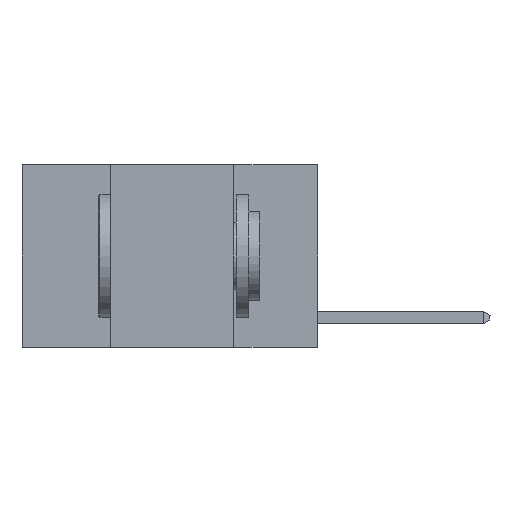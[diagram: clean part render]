
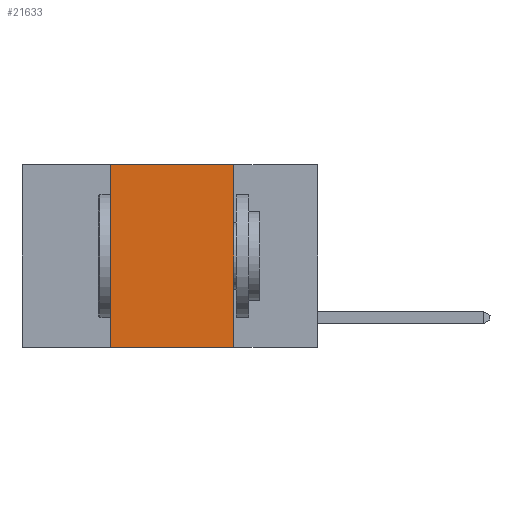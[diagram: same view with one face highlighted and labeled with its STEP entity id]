
A CAD part, left-side view. The second image highlights one B-rep face of the part: STEP entity #21633.
In plain terms, the highlighted planar face has unit normal (-1, 0, 0).
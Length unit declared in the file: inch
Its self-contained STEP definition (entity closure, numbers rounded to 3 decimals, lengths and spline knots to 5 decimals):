
#229 = CARTESIAN_POINT ( 'NONE',  ( 0., 0.17, 0. ) ) ;
#796 = DIRECTION ( 'NONE',  ( 1., 0., 0. ) ) ;
#931 = DIRECTION ( 'NONE',  ( 0., 0., -1. ) ) ;
#1075 = CARTESIAN_POINT ( 'NONE',  ( 0., 0.42, 0. ) ) ;
#3218 = CARTESIAN_POINT ( 'NONE',  ( 0., 0.17, -0.37 ) ) ;
#4366 = FACE_OUTER_BOUND ( 'NONE', #9969, .T. ) ;
#5682 = AXIS2_PLACEMENT_3D ( 'NONE', #17967, #796, #931 ) ;
#6763 = CARTESIAN_POINT ( 'NONE',  ( 0., 0.42, -0.37 ) ) ;
#7864 = CARTESIAN_POINT ( 'NONE',  ( 0., 0.42, 0. ) ) ;
#9466 = CARTESIAN_POINT ( 'NONE',  ( 0., 0.6, 0. ) ) ;
#9570 = EDGE_CURVE ( 'NONE', #17184, #23157, #17550, .T. ) ;
#9969 = EDGE_LOOP ( 'NONE', ( #13974, #13538, #19743, #16135 ) ) ;
#11245 = VECTOR ( 'NONE', #22871, 39.37008 ) ;
#11445 = DIRECTION ( 'NONE',  ( 0., 0., 1. ) ) ;
#12178 = LINE ( 'NONE', #13918, #15008 ) ;
#12338 = DIRECTION ( 'NONE',  ( 0., 0., -1. ) ) ;
#12817 = VERTEX_POINT ( 'NONE', #3218 ) ;
#13538 = ORIENTED_EDGE ( 'NONE', *, *, #23262, .F. ) ;
#13715 = EDGE_CURVE ( 'NONE', #22496, #12817, #23728, .T. ) ;
#13873 = PLANE ( 'NONE',  #5682 ) ;
#13918 = CARTESIAN_POINT ( 'NONE',  ( 0., 0.6, -0.37 ) ) ;
#13974 = ORIENTED_EDGE ( 'NONE', *, *, #13715, .F. ) ;
#15008 = VECTOR ( 'NONE', #21244, 39.37008 ) ;
#15680 = LINE ( 'NONE', #9466, #11245 ) ;
#15823 = VECTOR ( 'NONE', #12338, 39.37008 ) ;
#16135 = ORIENTED_EDGE ( 'NONE', *, *, #17335, .T. ) ;
#17184 = VERTEX_POINT ( 'NONE', #6763 ) ;
#17335 = EDGE_CURVE ( 'NONE', #17184, #12817, #12178, .T. ) ;
#17550 = LINE ( 'NONE', #7864, #23954 ) ;
#17967 = CARTESIAN_POINT ( 'NONE',  ( 0., 0.6, 0. ) ) ;
#18043 = CARTESIAN_POINT ( 'NONE',  ( 0., 0.17, 0. ) ) ;
#19743 = ORIENTED_EDGE ( 'NONE', *, *, #9570, .F. ) ;
#21244 = DIRECTION ( 'NONE',  ( 0., -1., 0. ) ) ;
#21633 = ADVANCED_FACE ( 'NONE', ( #4366 ), #13873, .F. ) ;
#22496 = VERTEX_POINT ( 'NONE', #229 ) ;
#22871 = DIRECTION ( 'NONE',  ( 0., -1., 0. ) ) ;
#23157 = VERTEX_POINT ( 'NONE', #1075 ) ;
#23262 = EDGE_CURVE ( 'NONE', #23157, #22496, #15680, .T. ) ;
#23728 = LINE ( 'NONE', #18043, #15823 ) ;
#23954 = VECTOR ( 'NONE', #11445, 39.37008 ) ;
